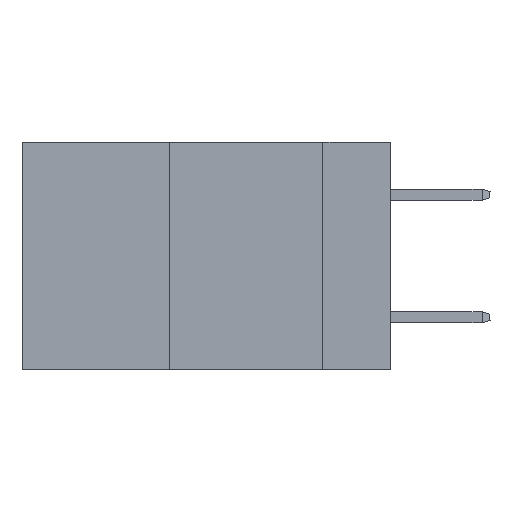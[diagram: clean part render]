
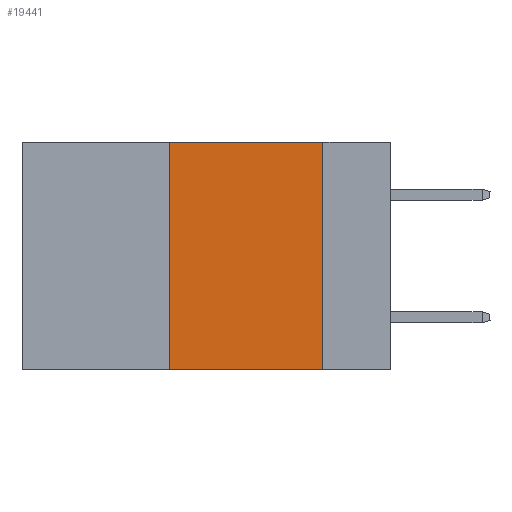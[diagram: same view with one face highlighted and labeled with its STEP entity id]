
A CAD part, left-side view. The second image highlights one B-rep face of the part: STEP entity #19441.
In plain terms, the highlighted planar face has unit normal (-1, 0, 0).
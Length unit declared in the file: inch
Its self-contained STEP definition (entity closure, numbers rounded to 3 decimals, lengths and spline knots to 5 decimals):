
#859 = DIRECTION ( 'NONE',  ( 0., 0., 1. ) ) ;
#1243 = DIRECTION ( 'NONE',  ( 0., -1., 0. ) ) ;
#2370 = EDGE_CURVE ( 'NONE', #25244, #12751, #18199, .T. ) ;
#2413 = VECTOR ( 'NONE', #859, 39.37008 ) ;
#5133 = EDGE_CURVE ( 'NONE', #31575, #19871, #28710, .T. ) ;
#5638 = CARTESIAN_POINT ( 'NONE',  ( 0., 0.6, 0. ) ) ;
#5757 = DIRECTION ( 'NONE',  ( 0., -1., 0. ) ) ;
#7485 = CARTESIAN_POINT ( 'NONE',  ( 0., 0.11, 0. ) ) ;
#9799 = ORIENTED_EDGE ( 'NONE', *, *, #33901, .F. ) ;
#11338 = CARTESIAN_POINT ( 'NONE',  ( 0., 0.36, -0.37 ) ) ;
#11750 = FACE_OUTER_BOUND ( 'NONE', #25870, .T. ) ;
#12751 = VERTEX_POINT ( 'NONE', #25192 ) ;
#15579 = VECTOR ( 'NONE', #5757, 39.37008 ) ;
#16417 = LINE ( 'NONE', #20957, #17273 ) ;
#17273 = VECTOR ( 'NONE', #1243, 39.37008 ) ;
#17395 = CARTESIAN_POINT ( 'NONE',  ( 0., 0.36, 0. ) ) ;
#18199 = LINE ( 'NONE', #17395, #2413 ) ;
#19441 = ADVANCED_FACE ( 'NONE', ( #11750 ), #21623, .F. ) ;
#19529 = ORIENTED_EDGE ( 'NONE', *, *, #5133, .F. ) ;
#19871 = VERTEX_POINT ( 'NONE', #31897 ) ;
#20957 = CARTESIAN_POINT ( 'NONE',  ( 0., 0.6, -0.37 ) ) ;
#21623 = PLANE ( 'NONE',  #23891 ) ;
#22168 = EDGE_CURVE ( 'NONE', #25244, #19871, #16417, .T. ) ;
#23891 = AXIS2_PLACEMENT_3D ( 'NONE', #24707, #24597, #30356 ) ;
#24573 = DIRECTION ( 'NONE',  ( 0., 0., -1. ) ) ;
#24597 = DIRECTION ( 'NONE',  ( 1., 0., 0. ) ) ;
#24707 = CARTESIAN_POINT ( 'NONE',  ( 0., 0.6, 0. ) ) ;
#25192 = CARTESIAN_POINT ( 'NONE',  ( 0., 0.36, 0. ) ) ;
#25244 = VERTEX_POINT ( 'NONE', #11338 ) ;
#25870 = EDGE_LOOP ( 'NONE', ( #19529, #9799, #32867, #27423 ) ) ;
#26929 = VECTOR ( 'NONE', #24573, 39.37008 ) ;
#27423 = ORIENTED_EDGE ( 'NONE', *, *, #22168, .T. ) ;
#28354 = LINE ( 'NONE', #5638, #15579 ) ;
#28710 = LINE ( 'NONE', #7485, #26929 ) ;
#30356 = DIRECTION ( 'NONE',  ( 0., 0., -1. ) ) ;
#31575 = VERTEX_POINT ( 'NONE', #32902 ) ;
#31897 = CARTESIAN_POINT ( 'NONE',  ( 0., 0.11, -0.37 ) ) ;
#32867 = ORIENTED_EDGE ( 'NONE', *, *, #2370, .F. ) ;
#32902 = CARTESIAN_POINT ( 'NONE',  ( 0., 0.11, 0. ) ) ;
#33901 = EDGE_CURVE ( 'NONE', #12751, #31575, #28354, .T. ) ;
